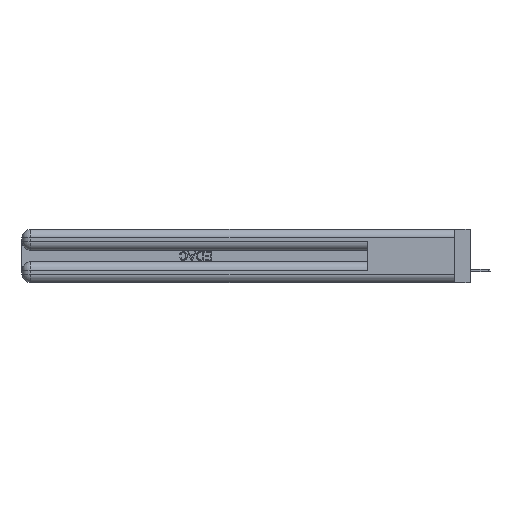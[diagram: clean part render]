
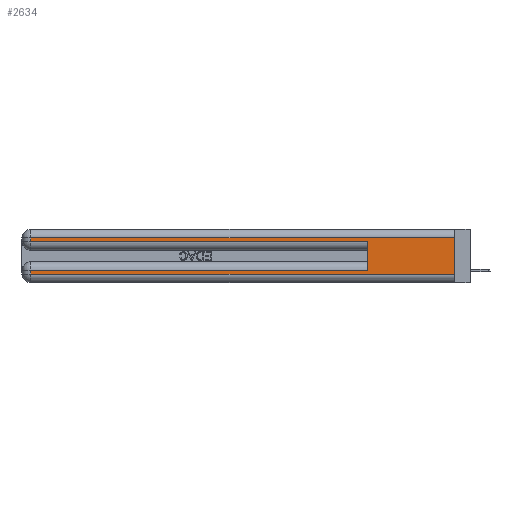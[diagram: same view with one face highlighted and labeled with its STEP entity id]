
A CAD part, left-side view. The second image highlights one B-rep face of the part: STEP entity #2634.
In plain terms, the highlighted planar face has unit normal (-1, 0, 0).
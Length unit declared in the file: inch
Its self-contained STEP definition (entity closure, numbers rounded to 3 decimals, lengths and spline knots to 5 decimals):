
#1107 = LINE ( 'NONE', #37439, #33085 ) ;
#1240 = DIRECTION ( 'NONE',  ( 1., 0., 0. ) ) ;
#2041 = CARTESIAN_POINT ( 'NONE',  ( 0., 2.94, 0.285 ) ) ;
#2634 = ADVANCED_FACE ( 'NONE', ( #37048 ), #33666, .F. ) ;
#3223 = CARTESIAN_POINT ( 'NONE',  ( 0., 0., 0.37 ) ) ;
#3807 = DIRECTION ( 'NONE',  ( 0., 0., 1. ) ) ;
#4013 = DIRECTION ( 'NONE',  ( 0., -1., 0. ) ) ;
#4497 = CARTESIAN_POINT ( 'NONE',  ( 0., 0., 0.285 ) ) ;
#4520 = VERTEX_POINT ( 'NONE', #31764 ) ;
#5336 = ORIENTED_EDGE ( 'NONE', *, *, #9334, .T. ) ;
#6960 = LINE ( 'NONE', #26661, #33402 ) ;
#7011 = EDGE_LOOP ( 'NONE', ( #40623, #8351, #31716, #30970, #18135, #35660, #5336, #35105 ) ) ;
#7747 = EDGE_CURVE ( 'NONE', #15731, #20979, #6960, .T. ) ;
#8137 = DIRECTION ( 'NONE',  ( 0., 1., 0. ) ) ;
#8351 = ORIENTED_EDGE ( 'NONE', *, *, #38223, .T. ) ;
#9136 = EDGE_CURVE ( 'NONE', #18101, #34004, #49371, .T. ) ;
#9148 = CARTESIAN_POINT ( 'NONE',  ( 0., 0., 0.06 ) ) ;
#9334 = EDGE_CURVE ( 'NONE', #14268, #9511, #1107, .T. ) ;
#9511 = VERTEX_POINT ( 'NONE', #25743 ) ;
#9548 = CARTESIAN_POINT ( 'NONE',  ( 0., 0., 0.37 ) ) ;
#11283 = LINE ( 'NONE', #3223, #27111 ) ;
#12520 = CARTESIAN_POINT ( 'NONE',  ( 0., 0., 0.31 ) ) ;
#13649 = DIRECTION ( 'NONE',  ( 0., 1., 0. ) ) ;
#14268 = VERTEX_POINT ( 'NONE', #31614 ) ;
#14902 = DIRECTION ( 'NONE',  ( 0., 0., -1. ) ) ;
#15731 = VERTEX_POINT ( 'NONE', #46100 ) ;
#16274 = EDGE_CURVE ( 'NONE', #9511, #19256, #27359, .T. ) ;
#17078 = DIRECTION ( 'NONE',  ( 0., 0., -1. ) ) ;
#17691 = EDGE_CURVE ( 'NONE', #4520, #19256, #11283, .T. ) ;
#18101 = VERTEX_POINT ( 'NONE', #49304 ) ;
#18135 = ORIENTED_EDGE ( 'NONE', *, *, #7747, .F. ) ;
#18311 = DIRECTION ( 'NONE',  ( 0., 0., -1. ) ) ;
#19256 = VERTEX_POINT ( 'NONE', #9148 ) ;
#20979 = VERTEX_POINT ( 'NONE', #23612 ) ;
#22376 = AXIS2_PLACEMENT_3D ( 'NONE', #9548, #1240, #17078 ) ;
#23612 = CARTESIAN_POINT ( 'NONE',  ( 0., 0.6, 0.285 ) ) ;
#25743 = CARTESIAN_POINT ( 'NONE',  ( 0., 2.94, 0.06 ) ) ;
#25809 = VECTOR ( 'NONE', #8137, 39.37008 ) ;
#26661 = CARTESIAN_POINT ( 'NONE',  ( 0., 0.6, 0.145 ) ) ;
#27111 = VECTOR ( 'NONE', #18311, 39.37008 ) ;
#27359 = LINE ( 'NONE', #35926, #33624 ) ;
#29102 = DIRECTION ( 'NONE',  ( 0., 0., -1. ) ) ;
#30132 = EDGE_CURVE ( 'NONE', #15731, #14268, #41157, .T. ) ;
#30970 = ORIENTED_EDGE ( 'NONE', *, *, #39436, .T. ) ;
#31383 = VECTOR ( 'NONE', #14902, 39.37008 ) ;
#31614 = CARTESIAN_POINT ( 'NONE',  ( 0., 2.94, 0.085 ) ) ;
#31716 = ORIENTED_EDGE ( 'NONE', *, *, #9136, .T. ) ;
#31764 = CARTESIAN_POINT ( 'NONE',  ( 0., 0., 0.31 ) ) ;
#33085 = VECTOR ( 'NONE', #29102, 39.37008 ) ;
#33402 = VECTOR ( 'NONE', #3807, 39.37008 ) ;
#33624 = VECTOR ( 'NONE', #4013, 39.37008 ) ;
#33666 = PLANE ( 'NONE',  #22376 ) ;
#34004 = VERTEX_POINT ( 'NONE', #2041 ) ;
#34139 = VECTOR ( 'NONE', #43934, 39.37008 ) ;
#35105 = ORIENTED_EDGE ( 'NONE', *, *, #16274, .T. ) ;
#35660 = ORIENTED_EDGE ( 'NONE', *, *, #30132, .T. ) ;
#35926 = CARTESIAN_POINT ( 'NONE',  ( 0., 0., 0.06 ) ) ;
#37048 = FACE_OUTER_BOUND ( 'NONE', #7011, .T. ) ;
#37439 = CARTESIAN_POINT ( 'NONE',  ( 0., 2.94, 0.37 ) ) ;
#38223 = EDGE_CURVE ( 'NONE', #4520, #18101, #40779, .T. ) ;
#39436 = EDGE_CURVE ( 'NONE', #34004, #20979, #48793, .T. ) ;
#40623 = ORIENTED_EDGE ( 'NONE', *, *, #17691, .F. ) ;
#40779 = LINE ( 'NONE', #12520, #25809 ) ;
#41157 = LINE ( 'NONE', #49169, #45857 ) ;
#43934 = DIRECTION ( 'NONE',  ( 0., -1., 0. ) ) ;
#45506 = CARTESIAN_POINT ( 'NONE',  ( 0., 2.94, 0.37 ) ) ;
#45857 = VECTOR ( 'NONE', #13649, 39.37008 ) ;
#46100 = CARTESIAN_POINT ( 'NONE',  ( 0., 0.6, 0.085 ) ) ;
#48793 = LINE ( 'NONE', #4497, #34139 ) ;
#49169 = CARTESIAN_POINT ( 'NONE',  ( 0., 0., 0.085 ) ) ;
#49304 = CARTESIAN_POINT ( 'NONE',  ( 0., 2.94, 0.31 ) ) ;
#49371 = LINE ( 'NONE', #45506, #31383 ) ;
